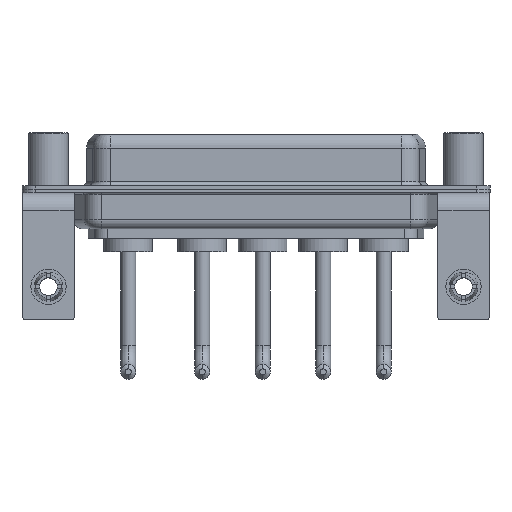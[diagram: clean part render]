
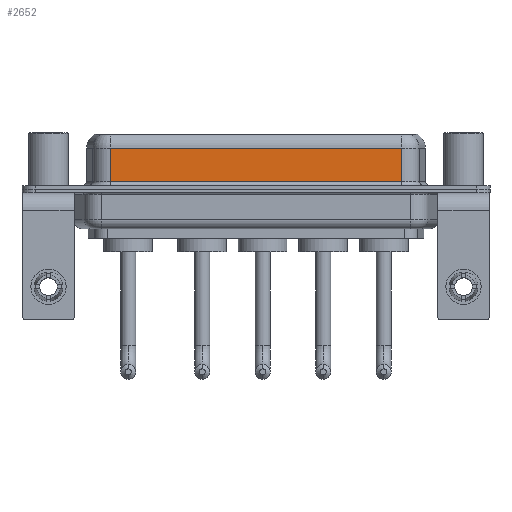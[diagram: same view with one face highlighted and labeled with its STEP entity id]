
A CAD part, front view. The second image highlights one B-rep face of the part: STEP entity #2652.
In plain terms, the highlighted planar face has unit normal (0, -1, 0).
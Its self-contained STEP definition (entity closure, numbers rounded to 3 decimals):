
#41 = VERTEX_POINT ( 'NONE', #3693 ) ;
#326 = DIRECTION ( 'NONE',  ( -1., 0., 0. ) ) ;
#387 = LINE ( 'NONE', #5410, #15532 ) ;
#2022 = DIRECTION ( 'NONE',  ( 0., 1., 0. ) ) ;
#2652 = ADVANCED_FACE ( 'NONE', ( #11558 ), #10347, .F. ) ;
#2846 = EDGE_CURVE ( 'NONE', #14377, #15247, #14931, .T. ) ;
#3230 = DIRECTION ( 'NONE',  ( 0., 0., -1. ) ) ;
#3662 = DIRECTION ( 'NONE',  ( 0., 0., -1. ) ) ;
#3693 = CARTESIAN_POINT ( 'NONE',  ( 40.037, -3.95, 0.9 ) ) ;
#4654 = VERTEX_POINT ( 'NONE', #12857 ) ;
#4774 = EDGE_CURVE ( 'NONE', #4654, #41, #15979, .T. ) ;
#5410 = CARTESIAN_POINT ( 'NONE',  ( 40.037, -3.95, 0.9 ) ) ;
#6694 = EDGE_LOOP ( 'NONE', ( #7384, #12273, #13413, #9407 ) ) ;
#7042 = VECTOR ( 'NONE', #3230, 1000. ) ;
#7384 = ORIENTED_EDGE ( 'NONE', *, *, #4774, .F. ) ;
#9407 = ORIENTED_EDGE ( 'NONE', *, *, #13906, .T. ) ;
#9502 = CARTESIAN_POINT ( 'NONE',  ( 40.037, -3.95, 6.4 ) ) ;
#10347 = PLANE ( 'NONE',  #12508 ) ;
#10976 = CARTESIAN_POINT ( 'NONE',  ( 7.013, -3.95, 6.4 ) ) ;
#11188 = VECTOR ( 'NONE', #3662, 1000. ) ;
#11343 = CARTESIAN_POINT ( 'NONE',  ( 40.037, -3.95, 4.65 ) ) ;
#11558 = FACE_OUTER_BOUND ( 'NONE', #6694, .T. ) ;
#11799 = DIRECTION ( 'NONE',  ( 0., 0., 1. ) ) ;
#11881 = CARTESIAN_POINT ( 'NONE',  ( 40.037, -3.95, 6.4 ) ) ;
#11968 = CARTESIAN_POINT ( 'NONE',  ( 7.013, -3.95, 4.65 ) ) ;
#11972 = EDGE_CURVE ( 'NONE', #4654, #14377, #12894, .T. ) ;
#12009 = CARTESIAN_POINT ( 'NONE',  ( 7.013, -3.95, 0.9 ) ) ;
#12273 = ORIENTED_EDGE ( 'NONE', *, *, #11972, .T. ) ;
#12508 = AXIS2_PLACEMENT_3D ( 'NONE', #11881, #2022, #11799 ) ;
#12857 = CARTESIAN_POINT ( 'NONE',  ( 40.037, -3.95, 4.65 ) ) ;
#12894 = LINE ( 'NONE', #11343, #14953 ) ;
#13413 = ORIENTED_EDGE ( 'NONE', *, *, #2846, .T. ) ;
#13906 = EDGE_CURVE ( 'NONE', #15247, #41, #387, .T. ) ;
#14377 = VERTEX_POINT ( 'NONE', #11968 ) ;
#14931 = LINE ( 'NONE', #10976, #11188 ) ;
#14953 = VECTOR ( 'NONE', #326, 1000. ) ;
#15247 = VERTEX_POINT ( 'NONE', #12009 ) ;
#15532 = VECTOR ( 'NONE', #15605, 1000. ) ;
#15605 = DIRECTION ( 'NONE',  ( 1., 0., 0. ) ) ;
#15979 = LINE ( 'NONE', #9502, #7042 ) ;
